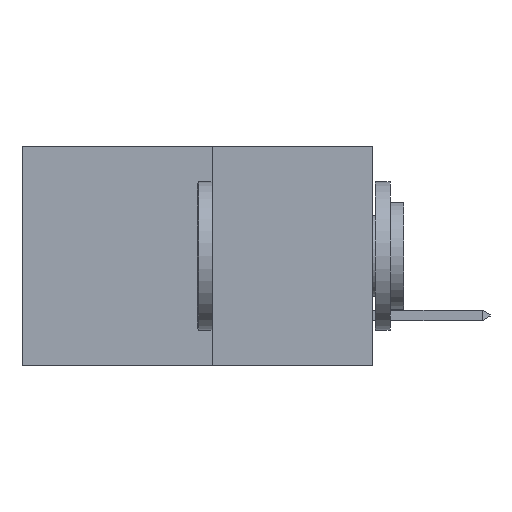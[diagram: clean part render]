
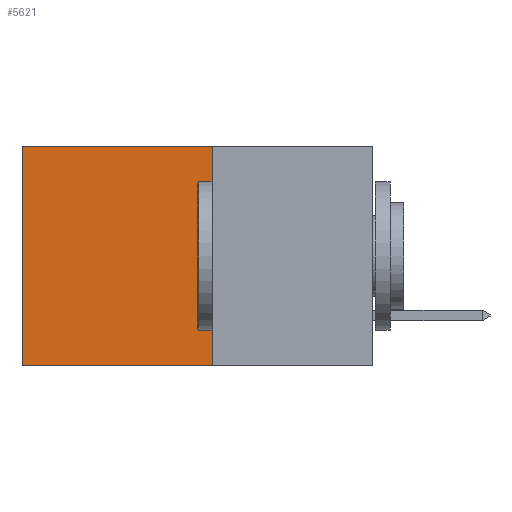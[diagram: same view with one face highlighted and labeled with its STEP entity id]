
A CAD part, left-side view. The second image highlights one B-rep face of the part: STEP entity #5621.
In plain terms, the highlighted planar face has unit normal (-1, 0, 0).
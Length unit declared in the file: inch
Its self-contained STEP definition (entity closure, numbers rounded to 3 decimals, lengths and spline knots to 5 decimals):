
#125 = LINE ( 'NONE', #2141, #10462 ) ;
#342 = EDGE_LOOP ( 'NONE', ( #8292, #7130, #12249, #5723 ) ) ;
#390 = CARTESIAN_POINT ( 'NONE',  ( 0.277, 0.27, -0.37 ) ) ;
#446 = CARTESIAN_POINT ( 'NONE',  ( 0.277, 0.27, 0. ) ) ;
#1127 = DIRECTION ( 'NONE',  ( 0., 0., -1. ) ) ;
#1180 = VERTEX_POINT ( 'NONE', #3089 ) ;
#2141 = CARTESIAN_POINT ( 'NONE',  ( 0.277, 0.59, -0.37 ) ) ;
#2154 = LINE ( 'NONE', #7582, #10081 ) ;
#2369 = DIRECTION ( 'NONE',  ( 0., 1., 0. ) ) ;
#3089 = CARTESIAN_POINT ( 'NONE',  ( 0.277, 0.59, 0. ) ) ;
#3436 = VECTOR ( 'NONE', #11296, 39.37008 ) ;
#3470 = EDGE_CURVE ( 'NONE', #10420, #1180, #11325, .T. ) ;
#4087 = LINE ( 'NONE', #11687, #11959 ) ;
#4424 = FACE_OUTER_BOUND ( 'NONE', #342, .T. ) ;
#5500 = AXIS2_PLACEMENT_3D ( 'NONE', #11485, #11411, #11364 ) ;
#5621 = ADVANCED_FACE ( 'NONE', ( #4424 ), #11453, .F. ) ;
#5631 = EDGE_CURVE ( 'NONE', #10420, #11012, #4087, .T. ) ;
#5723 = ORIENTED_EDGE ( 'NONE', *, *, #3470, .T. ) ;
#6001 = EDGE_CURVE ( 'NONE', #11012, #11282, #2154, .T. ) ;
#7130 = ORIENTED_EDGE ( 'NONE', *, *, #6001, .F. ) ;
#7582 = CARTESIAN_POINT ( 'NONE',  ( 0.277, 0.27, -0.37 ) ) ;
#8292 = ORIENTED_EDGE ( 'NONE', *, *, #11495, .T. ) ;
#10081 = VECTOR ( 'NONE', #2369, 39.37008 ) ;
#10420 = VERTEX_POINT ( 'NONE', #446 ) ;
#10462 = VECTOR ( 'NONE', #1127, 39.37008 ) ;
#11012 = VERTEX_POINT ( 'NONE', #390 ) ;
#11197 = CARTESIAN_POINT ( 'NONE',  ( 0.277, 0.27, 0. ) ) ;
#11282 = VERTEX_POINT ( 'NONE', #12127 ) ;
#11296 = DIRECTION ( 'NONE',  ( 0., 1., 0. ) ) ;
#11325 = LINE ( 'NONE', #11197, #3436 ) ;
#11364 = DIRECTION ( 'NONE',  ( 0., 0., -1. ) ) ;
#11411 = DIRECTION ( 'NONE',  ( 1., 0., 0. ) ) ;
#11453 = PLANE ( 'NONE',  #5500 ) ;
#11485 = CARTESIAN_POINT ( 'NONE',  ( 0.277, 0.27, -0.37 ) ) ;
#11495 = EDGE_CURVE ( 'NONE', #1180, #11282, #125, .T. ) ;
#11666 = DIRECTION ( 'NONE',  ( 0., 0., -1. ) ) ;
#11687 = CARTESIAN_POINT ( 'NONE',  ( 0.277, 0.27, -0.37 ) ) ;
#11959 = VECTOR ( 'NONE', #11666, 39.37008 ) ;
#12127 = CARTESIAN_POINT ( 'NONE',  ( 0.277, 0.59, -0.37 ) ) ;
#12249 = ORIENTED_EDGE ( 'NONE', *, *, #5631, .F. ) ;
